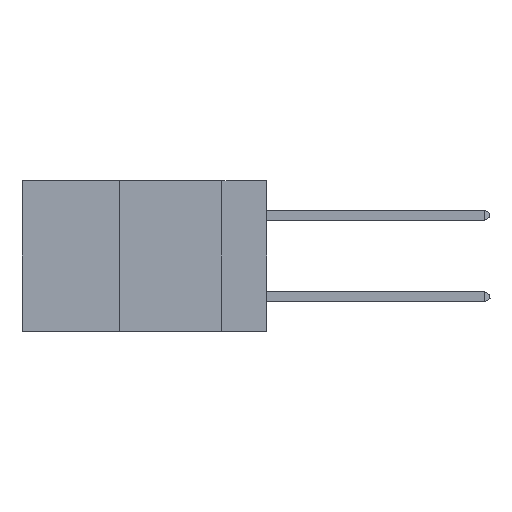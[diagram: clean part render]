
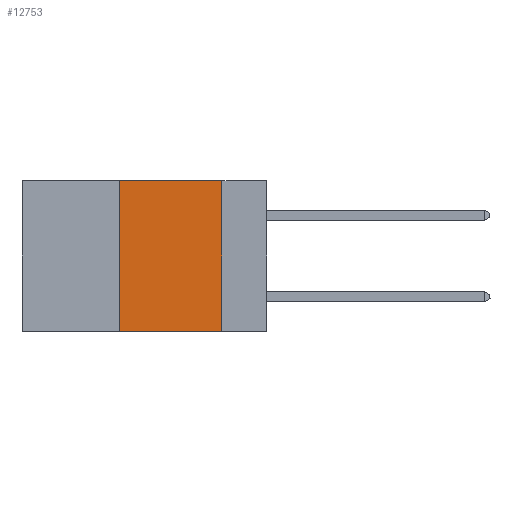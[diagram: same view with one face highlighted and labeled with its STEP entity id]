
A CAD part, left-side view. The second image highlights one B-rep face of the part: STEP entity #12753.
In plain terms, the highlighted planar face has unit normal (-1, 0, 0).
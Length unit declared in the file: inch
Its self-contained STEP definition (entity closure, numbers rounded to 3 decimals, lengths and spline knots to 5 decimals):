
#2193 = VECTOR ( 'NONE', #8711, 39.37008 ) ;
#2482 = LINE ( 'NONE', #4735, #2193 ) ;
#3825 = CARTESIAN_POINT ( 'NONE',  ( 0., 0.11, 0. ) ) ;
#3935 = DIRECTION ( 'NONE',  ( 1., 0., 0. ) ) ;
#4516 = VERTEX_POINT ( 'NONE', #3825 ) ;
#4735 = CARTESIAN_POINT ( 'NONE',  ( 0., 0.36, 0. ) ) ;
#5491 = ORIENTED_EDGE ( 'NONE', *, *, #17822, .F. ) ;
#7821 = CARTESIAN_POINT ( 'NONE',  ( 0., 0.6, 0. ) ) ;
#8043 = ORIENTED_EDGE ( 'NONE', *, *, #9495, .F. ) ;
#8392 = VERTEX_POINT ( 'NONE', #11347 ) ;
#8711 = DIRECTION ( 'NONE',  ( 0., 0., 1. ) ) ;
#9495 = EDGE_CURVE ( 'NONE', #8392, #4516, #20715, .T. ) ;
#9963 = VECTOR ( 'NONE', #46256, 39.37008 ) ;
#10067 = LINE ( 'NONE', #42895, #9963 ) ;
#11347 = CARTESIAN_POINT ( 'NONE',  ( 0., 0.36, 0. ) ) ;
#11741 = DIRECTION ( 'NONE',  ( 0., -1., 0. ) ) ;
#12753 = ADVANCED_FACE ( 'NONE', ( #29839 ), #26563, .F. ) ;
#14605 = EDGE_CURVE ( 'NONE', #40969, #27530, #10067, .T. ) ;
#15444 = EDGE_CURVE ( 'NONE', #40969, #8392, #2482, .T. ) ;
#16000 = VECTOR ( 'NONE', #23158, 39.37008 ) ;
#16042 = LINE ( 'NONE', #29990, #16000 ) ;
#17822 = EDGE_CURVE ( 'NONE', #4516, #27530, #16042, .T. ) ;
#19050 = AXIS2_PLACEMENT_3D ( 'NONE', #36750, #3935, #30036 ) ;
#20464 = VECTOR ( 'NONE', #11741, 39.37008 ) ;
#20715 = LINE ( 'NONE', #7821, #20464 ) ;
#23158 = DIRECTION ( 'NONE',  ( 0., 0., -1. ) ) ;
#26563 = PLANE ( 'NONE',  #19050 ) ;
#27530 = VERTEX_POINT ( 'NONE', #36583 ) ;
#29839 = FACE_OUTER_BOUND ( 'NONE', #31853, .T. ) ;
#29990 = CARTESIAN_POINT ( 'NONE',  ( 0., 0.11, 0. ) ) ;
#30036 = DIRECTION ( 'NONE',  ( 0., 0., -1. ) ) ;
#31853 = EDGE_LOOP ( 'NONE', ( #5491, #8043, #32470, #34442 ) ) ;
#32470 = ORIENTED_EDGE ( 'NONE', *, *, #15444, .F. ) ;
#34442 = ORIENTED_EDGE ( 'NONE', *, *, #14605, .T. ) ;
#36583 = CARTESIAN_POINT ( 'NONE',  ( 0., 0.11, -0.37 ) ) ;
#36750 = CARTESIAN_POINT ( 'NONE',  ( 0., 0.6, 0. ) ) ;
#40969 = VERTEX_POINT ( 'NONE', #42374 ) ;
#42374 = CARTESIAN_POINT ( 'NONE',  ( 0., 0.36, -0.37 ) ) ;
#42895 = CARTESIAN_POINT ( 'NONE',  ( 0., 0.6, -0.37 ) ) ;
#46256 = DIRECTION ( 'NONE',  ( 0., -1., 0. ) ) ;
